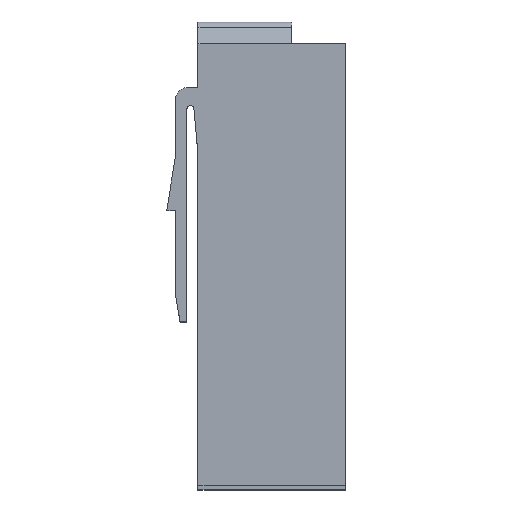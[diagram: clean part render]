
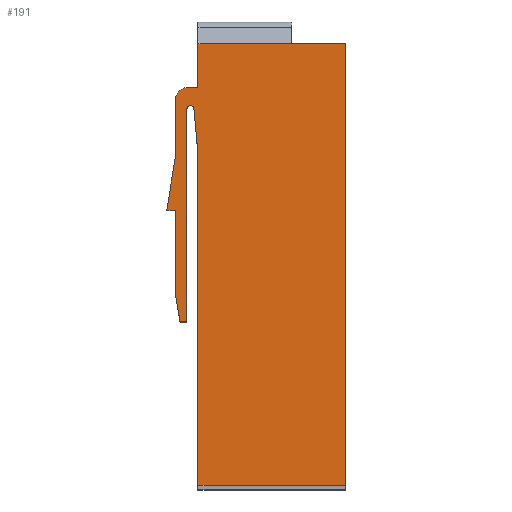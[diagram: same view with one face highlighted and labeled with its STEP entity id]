
A CAD part, top view. The second image highlights one B-rep face of the part: STEP entity #191.
In plain terms, the highlighted planar face has unit normal (0, 0, 1).
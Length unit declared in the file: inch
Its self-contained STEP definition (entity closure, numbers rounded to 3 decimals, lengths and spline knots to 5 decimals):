
#16 = LINE ( 'NONE', #659, #846 ) ;
#25 = CARTESIAN_POINT ( 'NONE',  ( -0.19725, 4.28613, 0.75 ) ) ;
#28 = VERTEX_POINT ( 'NONE', #663 ) ;
#35 = DIRECTION ( 'NONE',  ( -1., 0., 0. ) ) ;
#38 = LINE ( 'NONE', #763, #611 ) ;
#73 = AXIS2_PLACEMENT_3D ( 'NONE', #579, #1125, #87 ) ;
#78 = VERTEX_POINT ( 'NONE', #25 ) ;
#79 = PLANE ( 'NONE',  #73 ) ;
#87 = DIRECTION ( 'NONE',  ( -1., 0., 0. ) ) ;
#90 = DIRECTION ( 'NONE',  ( 1., 0., 0. ) ) ;
#95 = VECTOR ( 'NONE', #1017, 39.37008 ) ;
#109 = ORIENTED_EDGE ( 'NONE', *, *, #1097, .F. ) ;
#110 = ORIENTED_EDGE ( 'NONE', *, *, #1107, .T. ) ;
#126 = ORIENTED_EDGE ( 'NONE', *, *, #1322, .F. ) ;
#148 = VECTOR ( 'NONE', #243, 39.37008 ) ;
#149 = AXIS2_PLACEMENT_3D ( 'NONE', #1197, #357, #239 ) ;
#157 = EDGE_CURVE ( 'NONE', #1316, #890, #1003, .T. ) ;
#173 = ORIENTED_EDGE ( 'NONE', *, *, #990, .F. ) ;
#180 = CARTESIAN_POINT ( 'NONE',  ( -0.275, 4.26496, 0.75 ) ) ;
#181 = LINE ( 'NONE', #323, #148 ) ;
#182 = DIRECTION ( 'NONE',  ( 0., 0., -1. ) ) ;
#183 = VECTOR ( 'NONE', #1339, 39.37008 ) ;
#191 = ADVANCED_FACE ( 'NONE', ( #988 ), #79, .F. ) ;
#200 = EDGE_CURVE ( 'NONE', #415, #1193, #733, .T. ) ;
#210 = ORIENTED_EDGE ( 'NONE', *, *, #200, .T. ) ;
#212 = DIRECTION ( 'NONE',  ( 0., -1., 0. ) ) ;
#213 = LINE ( 'NONE', #709, #471 ) ;
#236 = ORIENTED_EDGE ( 'NONE', *, *, #924, .T. ) ;
#237 = CARTESIAN_POINT ( 'NONE',  ( -0.4, 0., 0.75 ) ) ;
#239 = DIRECTION ( 'NONE',  ( 1., 0., 0. ) ) ;
#240 = VERTEX_POINT ( 'NONE', #180 ) ;
#243 = DIRECTION ( 'NONE',  ( 0.09, -0.996, 0. ) ) ;
#258 = EDGE_CURVE ( 'NONE', #396, #837, #1205, .T. ) ;
#273 = DIRECTION ( 'NONE',  ( 0., -1., 0. ) ) ;
#277 = LINE ( 'NONE', #1293, #487 ) ;
#294 = DIRECTION ( 'NONE',  ( 1., 0., 0. ) ) ;
#300 = ORIENTED_EDGE ( 'NONE', *, *, #1294, .F. ) ;
#304 = CARTESIAN_POINT ( 'NONE',  ( -0.275, 1.88125, 0.75 ) ) ;
#306 = EDGE_CURVE ( 'NONE', #1317, #769, #781, .T. ) ;
#323 = CARTESIAN_POINT ( 'NONE',  ( 0.18795, 0.01696, 0.75 ) ) ;
#344 = CARTESIAN_POINT ( 'NONE',  ( -0.15, 0.05, 0.75 ) ) ;
#357 = DIRECTION ( 'NONE',  ( 0., 0., -1. ) ) ;
#362 = ORIENTED_EDGE ( 'NONE', *, *, #824, .T. ) ;
#365 = CARTESIAN_POINT ( 'NONE',  ( 0., 5., 0.75 ) ) ;
#388 = CARTESIAN_POINT ( 'NONE',  ( -0.23306, 4.2643, 0.75 ) ) ;
#396 = VERTEX_POINT ( 'NONE', #608 ) ;
#405 = DIRECTION ( 'NONE',  ( 0., -1., 0. ) ) ;
#415 = VERTEX_POINT ( 'NONE', #722 ) ;
#428 = ORIENTED_EDGE ( 'NONE', *, *, #646, .T. ) ;
#440 = CIRCLE ( 'NONE', #636, 0.04194 ) ;
#447 = DIRECTION ( 'NONE',  ( 1., 0., 0. ) ) ;
#462 = CARTESIAN_POINT ( 'NONE',  ( -0.35, 1.88125, 0.75 ) ) ;
#471 = VECTOR ( 'NONE', #405, 39.37008 ) ;
#477 = VERTEX_POINT ( 'NONE', #618 ) ;
#484 = ORIENTED_EDGE ( 'NONE', *, *, #157, .T. ) ;
#487 = VECTOR ( 'NONE', #35, 39.37008 ) ;
#495 = CARTESIAN_POINT ( 'NONE',  ( -0.15, 5., 0.75 ) ) ;
#518 = CARTESIAN_POINT ( 'NONE',  ( 0., 4.50625, 0.75 ) ) ;
#551 = CARTESIAN_POINT ( 'NONE',  ( -0.4, 2.16481, 0.75 ) ) ;
#579 = CARTESIAN_POINT ( 'NONE',  ( 0., 5., 0.75 ) ) ;
#589 = ORIENTED_EDGE ( 'NONE', *, *, #843, .T. ) ;
#608 = CARTESIAN_POINT ( 'NONE',  ( 1.5, 5., 0.75 ) ) ;
#611 = VECTOR ( 'NONE', #1301, 39.37008 ) ;
#618 = CARTESIAN_POINT ( 'NONE',  ( -0.15, 3.7625, 0.75 ) ) ;
#635 = ORIENTED_EDGE ( 'NONE', *, *, #945, .T. ) ;
#636 = AXIS2_PLACEMENT_3D ( 'NONE', #388, #182, #294 ) ;
#646 = EDGE_CURVE ( 'NONE', #890, #415, #38, .T. ) ;
#648 = LINE ( 'NONE', #365, #1000 ) ;
#659 = CARTESIAN_POINT ( 'NONE',  ( 0., 5., 0.75 ) ) ;
#663 = CARTESIAN_POINT ( 'NONE',  ( -0.15, 4.50625, 0.75 ) ) ;
#709 = CARTESIAN_POINT ( 'NONE',  ( -0.275, 0., 0.75 ) ) ;
#712 = VECTOR ( 'NONE', #273, 39.37008 ) ;
#722 = CARTESIAN_POINT ( 'NONE',  ( -0.5, 3.13125, 0.75 ) ) ;
#724 = CARTESIAN_POINT ( 'NONE',  ( -0.4, 0., 0.75 ) ) ;
#729 = DIRECTION ( 'NONE',  ( 1., 0., 0. ) ) ;
#733 = LINE ( 'NONE', #1330, #1219 ) ;
#739 = CARTESIAN_POINT ( 'NONE',  ( -0.4, 3.13125, 0.75 ) ) ;
#754 = ORIENTED_EDGE ( 'NONE', *, *, #1280, .F. ) ;
#761 = LINE ( 'NONE', #724, #1327 ) ;
#763 = CARTESIAN_POINT ( 'NONE',  ( -0.97601, 0.15616, 0.75 ) ) ;
#769 = VERTEX_POINT ( 'NONE', #462 ) ;
#775 = EDGE_CURVE ( 'NONE', #940, #396, #648, .T. ) ;
#781 = LINE ( 'NONE', #1336, #1286 ) ;
#786 = ORIENTED_EDGE ( 'NONE', *, *, #306, .T. ) ;
#793 = LINE ( 'NONE', #1333, #1018 ) ;
#805 = CARTESIAN_POINT ( 'NONE',  ( 1.5, 0.05, 0.75 ) ) ;
#808 = DIRECTION ( 'NONE',  ( 0., -1., 0. ) ) ;
#813 = LINE ( 'NONE', #1026, #183 ) ;
#824 = EDGE_CURVE ( 'NONE', #477, #1306, #984, .T. ) ;
#837 = VERTEX_POINT ( 'NONE', #805 ) ;
#843 = EDGE_CURVE ( 'NONE', #240, #78, #440, .T. ) ;
#846 = VECTOR ( 'NONE', #447, 39.37008 ) ;
#854 = VERTEX_POINT ( 'NONE', #495 ) ;
#859 = EDGE_LOOP ( 'NONE', ( #110, #786, #635, #173, #589, #1224, #362, #300, #1332, #1060, #754, #236, #109, #126, #484, #428, #210 ) ) ;
#890 = VERTEX_POINT ( 'NONE', #1014 ) ;
#911 = DIRECTION ( 'NONE',  ( 1., 0., 0. ) ) ;
#917 = CARTESIAN_POINT ( 'NONE',  ( 1.5, 5., 0.75 ) ) ;
#924 = EDGE_CURVE ( 'NONE', #854, #28, #813, .T. ) ;
#930 = CIRCLE ( 'NONE', #149, 0.125 ) ;
#940 = VERTEX_POINT ( 'NONE', #1011 ) ;
#945 = EDGE_CURVE ( 'NONE', #769, #992, #793, .T. ) ;
#984 = LINE ( 'NONE', #993, #712 ) ;
#988 = FACE_OUTER_BOUND ( 'NONE', #859, .T. ) ;
#990 = EDGE_CURVE ( 'NONE', #240, #992, #213, .T. ) ;
#991 = CARTESIAN_POINT ( 'NONE',  ( -0.4, 4.38125, 0.75 ) ) ;
#992 = VERTEX_POINT ( 'NONE', #304 ) ;
#993 = CARTESIAN_POINT ( 'NONE',  ( -0.15, 5., 0.75 ) ) ;
#1000 = VECTOR ( 'NONE', #1216, 39.37008 ) ;
#1003 = LINE ( 'NONE', #237, #1315 ) ;
#1006 = DIRECTION ( 'NONE',  ( 0.174, -0.985, 0. ) ) ;
#1011 = CARTESIAN_POINT ( 'NONE',  ( 0.9, 5., 0.75 ) ) ;
#1014 = CARTESIAN_POINT ( 'NONE',  ( -0.4, 3.75625, 0.75 ) ) ;
#1017 = DIRECTION ( 'NONE',  ( 0., -1., 0. ) ) ;
#1018 = VECTOR ( 'NONE', #90, 39.37008 ) ;
#1026 = CARTESIAN_POINT ( 'NONE',  ( -0.15, 5., 0.75 ) ) ;
#1060 = ORIENTED_EDGE ( 'NONE', *, *, #775, .F. ) ;
#1062 = CARTESIAN_POINT ( 'NONE',  ( -0.275, 4.50625, 0.75 ) ) ;
#1097 = EDGE_CURVE ( 'NONE', #1210, #28, #1165, .T. ) ;
#1107 = EDGE_CURVE ( 'NONE', #1193, #1317, #761, .T. ) ;
#1125 = DIRECTION ( 'NONE',  ( 0., 0., -1. ) ) ;
#1148 = VECTOR ( 'NONE', #729, 39.37008 ) ;
#1165 = LINE ( 'NONE', #518, #1148 ) ;
#1193 = VERTEX_POINT ( 'NONE', #739 ) ;
#1197 = CARTESIAN_POINT ( 'NONE',  ( -0.275, 4.38125, 0.75 ) ) ;
#1205 = LINE ( 'NONE', #917, #95 ) ;
#1210 = VERTEX_POINT ( 'NONE', #1062 ) ;
#1216 = DIRECTION ( 'NONE',  ( 1., 0., 0. ) ) ;
#1219 = VECTOR ( 'NONE', #911, 39.37008 ) ;
#1222 = EDGE_CURVE ( 'NONE', #78, #477, #181, .T. ) ;
#1224 = ORIENTED_EDGE ( 'NONE', *, *, #1222, .T. ) ;
#1280 = EDGE_CURVE ( 'NONE', #854, #940, #16, .T. ) ;
#1286 = VECTOR ( 'NONE', #1006, 39.37008 ) ;
#1293 = CARTESIAN_POINT ( 'NONE',  ( 1.5, 0.05, 0.75 ) ) ;
#1294 = EDGE_CURVE ( 'NONE', #837, #1306, #277, .T. ) ;
#1301 = DIRECTION ( 'NONE',  ( -0.158, -0.987, 0. ) ) ;
#1306 = VERTEX_POINT ( 'NONE', #344 ) ;
#1315 = VECTOR ( 'NONE', #808, 39.37008 ) ;
#1316 = VERTEX_POINT ( 'NONE', #991 ) ;
#1317 = VERTEX_POINT ( 'NONE', #551 ) ;
#1322 = EDGE_CURVE ( 'NONE', #1316, #1210, #930, .T. ) ;
#1327 = VECTOR ( 'NONE', #212, 39.37008 ) ;
#1330 = CARTESIAN_POINT ( 'NONE',  ( 0., 3.13125, 0.75 ) ) ;
#1332 = ORIENTED_EDGE ( 'NONE', *, *, #258, .F. ) ;
#1333 = CARTESIAN_POINT ( 'NONE',  ( 0., 1.88125, 0.75 ) ) ;
#1336 = CARTESIAN_POINT ( 'NONE',  ( -0.4, 2.16481, 0.75 ) ) ;
#1339 = DIRECTION ( 'NONE',  ( 0., -1., 0. ) ) ;
